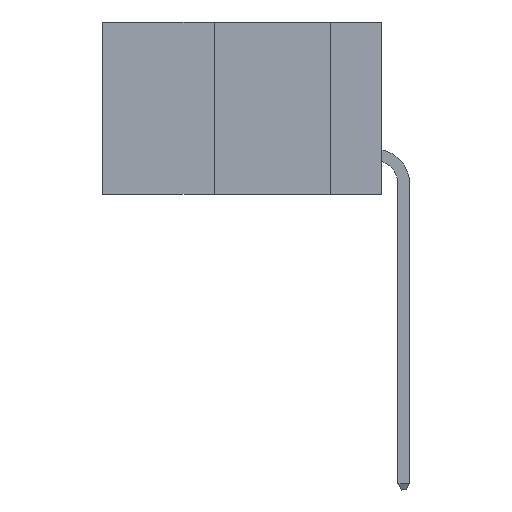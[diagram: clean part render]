
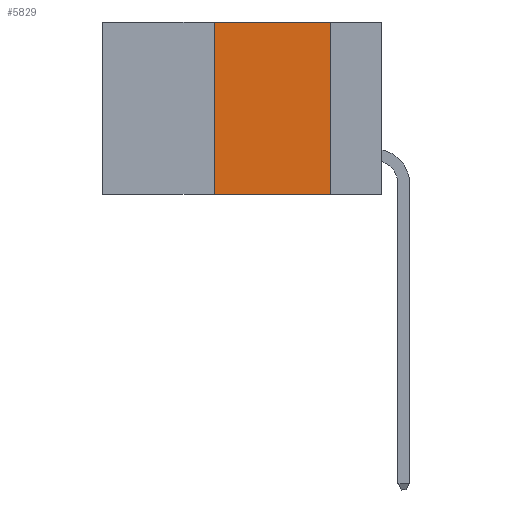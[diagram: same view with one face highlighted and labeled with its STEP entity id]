
A CAD part, left-side view. The second image highlights one B-rep face of the part: STEP entity #5829.
In plain terms, the highlighted planar face has unit normal (-1, 0, 0).
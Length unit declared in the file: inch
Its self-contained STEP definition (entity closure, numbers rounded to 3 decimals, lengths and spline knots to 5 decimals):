
#51 = VERTEX_POINT ( 'NONE', #1699 ) ;
#523 = CARTESIAN_POINT ( 'NONE',  ( 0., 0.36, 0. ) ) ;
#1074 = LINE ( 'NONE', #11516, #6848 ) ;
#1084 = VECTOR ( 'NONE', #11641, 39.37008 ) ;
#1699 = CARTESIAN_POINT ( 'NONE',  ( 0., 0.36, -0.37 ) ) ;
#1975 = ORIENTED_EDGE ( 'NONE', *, *, #4112, .F. ) ;
#2846 = DIRECTION ( 'NONE',  ( 0., 0., -1. ) ) ;
#3332 = VERTEX_POINT ( 'NONE', #523 ) ;
#4112 = EDGE_CURVE ( 'NONE', #3332, #5174, #13010, .T. ) ;
#4710 = ORIENTED_EDGE ( 'NONE', *, *, #5569, .F. ) ;
#4875 = VERTEX_POINT ( 'NONE', #13631 ) ;
#5174 = VERTEX_POINT ( 'NONE', #11566 ) ;
#5182 = EDGE_CURVE ( 'NONE', #51, #4875, #1074, .T. ) ;
#5569 = EDGE_CURVE ( 'NONE', #51, #3332, #11455, .T. ) ;
#5829 = ADVANCED_FACE ( 'NONE', ( #7313 ), #7509, .F. ) ;
#6848 = VECTOR ( 'NONE', #11570, 39.37008 ) ;
#7313 = FACE_OUTER_BOUND ( 'NONE', #10290, .T. ) ;
#7485 = DIRECTION ( 'NONE',  ( 0., 0., -1. ) ) ;
#7506 = DIRECTION ( 'NONE',  ( 1., 0., 0. ) ) ;
#7509 = PLANE ( 'NONE',  #8991 ) ;
#7729 = CARTESIAN_POINT ( 'NONE',  ( 0., 0.6, 0. ) ) ;
#7873 = VECTOR ( 'NONE', #8979, 39.37008 ) ;
#8348 = ORIENTED_EDGE ( 'NONE', *, *, #13877, .F. ) ;
#8699 = VECTOR ( 'NONE', #2846, 39.37008 ) ;
#8979 = DIRECTION ( 'NONE',  ( 0., 0., 1. ) ) ;
#8991 = AXIS2_PLACEMENT_3D ( 'NONE', #7729, #7506, #7485 ) ;
#8995 = CARTESIAN_POINT ( 'NONE',  ( 0., 0.36, 0. ) ) ;
#10290 = EDGE_LOOP ( 'NONE', ( #8348, #1975, #4710, #12786 ) ) ;
#10642 = CARTESIAN_POINT ( 'NONE',  ( 0., 0.11, 0. ) ) ;
#11455 = LINE ( 'NONE', #8995, #7873 ) ;
#11516 = CARTESIAN_POINT ( 'NONE',  ( 0., 0.6, -0.37 ) ) ;
#11566 = CARTESIAN_POINT ( 'NONE',  ( 0., 0.11, 0. ) ) ;
#11570 = DIRECTION ( 'NONE',  ( 0., -1., 0. ) ) ;
#11620 = LINE ( 'NONE', #10642, #8699 ) ;
#11641 = DIRECTION ( 'NONE',  ( 0., -1., 0. ) ) ;
#11655 = CARTESIAN_POINT ( 'NONE',  ( 0., 0.6, 0. ) ) ;
#12786 = ORIENTED_EDGE ( 'NONE', *, *, #5182, .T. ) ;
#13010 = LINE ( 'NONE', #11655, #1084 ) ;
#13631 = CARTESIAN_POINT ( 'NONE',  ( 0., 0.11, -0.37 ) ) ;
#13877 = EDGE_CURVE ( 'NONE', #5174, #4875, #11620, .T. ) ;
